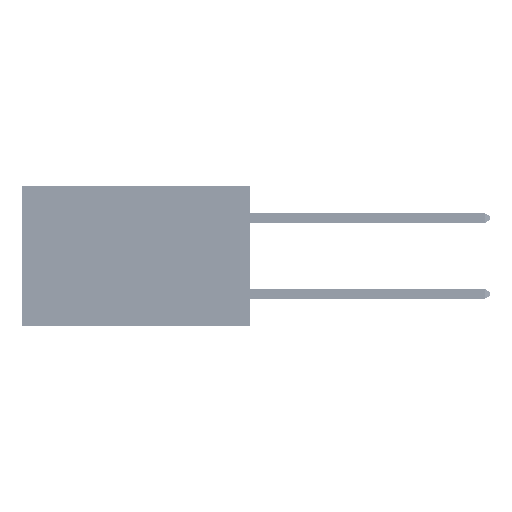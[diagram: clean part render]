
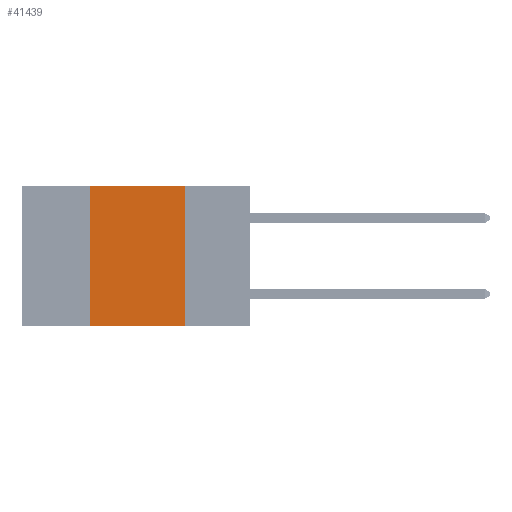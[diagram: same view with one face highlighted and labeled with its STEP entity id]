
A CAD part, left-side view. The second image highlights one B-rep face of the part: STEP entity #41439.
In plain terms, the highlighted planar face has unit normal (-1, 0, 0).
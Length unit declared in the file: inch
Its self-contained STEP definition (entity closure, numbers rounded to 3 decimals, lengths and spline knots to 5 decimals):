
#1589 = VECTOR ( 'NONE', #28482, 39.37008 ) ;
#3840 = VECTOR ( 'NONE', #15682, 39.37008 ) ;
#4211 = EDGE_CURVE ( 'NONE', #22656, #34241, #32235, .T. ) ;
#6393 = ORIENTED_EDGE ( 'NONE', *, *, #17723, .F. ) ;
#6564 = CARTESIAN_POINT ( 'NONE',  ( 0., 0.42, 0. ) ) ;
#7036 = DIRECTION ( 'NONE',  ( 1., 0., 0. ) ) ;
#7541 = ORIENTED_EDGE ( 'NONE', *, *, #4211, .T. ) ;
#10291 = EDGE_LOOP ( 'NONE', ( #6393, #43165, #33677, #7541 ) ) ;
#10614 = VECTOR ( 'NONE', #27359, 39.37008 ) ;
#14806 = CARTESIAN_POINT ( 'NONE',  ( 0., 0.6, -0.37 ) ) ;
#14842 = VECTOR ( 'NONE', #29393, 39.37008 ) ;
#15682 = DIRECTION ( 'NONE',  ( 0., -1., 0. ) ) ;
#17723 = EDGE_CURVE ( 'NONE', #29060, #34241, #45265, .T. ) ;
#19779 = CARTESIAN_POINT ( 'NONE',  ( 0., 0.42, 0. ) ) ;
#22656 = VERTEX_POINT ( 'NONE', #39769 ) ;
#24455 = CARTESIAN_POINT ( 'NONE',  ( 0., 0.6, 0. ) ) ;
#24463 = LINE ( 'NONE', #6564, #1589 ) ;
#25095 = VERTEX_POINT ( 'NONE', #19779 ) ;
#27359 = DIRECTION ( 'NONE',  ( 0., 0., -1. ) ) ;
#28482 = DIRECTION ( 'NONE',  ( 0., 0., 1. ) ) ;
#29060 = VERTEX_POINT ( 'NONE', #42988 ) ;
#29393 = DIRECTION ( 'NONE',  ( 0., -1., 0. ) ) ;
#29553 = CARTESIAN_POINT ( 'NONE',  ( 0., 0.17, -0.37 ) ) ;
#32235 = LINE ( 'NONE', #14806, #14842 ) ;
#32624 = EDGE_CURVE ( 'NONE', #25095, #29060, #41134, .T. ) ;
#33677 = ORIENTED_EDGE ( 'NONE', *, *, #39256, .F. ) ;
#34241 = VERTEX_POINT ( 'NONE', #29553 ) ;
#35774 = DIRECTION ( 'NONE',  ( 0., 0., -1. ) ) ;
#37142 = CARTESIAN_POINT ( 'NONE',  ( 0., 0.6, 0. ) ) ;
#38415 = CARTESIAN_POINT ( 'NONE',  ( 0., 0.17, 0. ) ) ;
#39245 = AXIS2_PLACEMENT_3D ( 'NONE', #24455, #7036, #35774 ) ;
#39256 = EDGE_CURVE ( 'NONE', #22656, #25095, #24463, .T. ) ;
#39769 = CARTESIAN_POINT ( 'NONE',  ( 0., 0.42, -0.37 ) ) ;
#41134 = LINE ( 'NONE', #37142, #3840 ) ;
#41439 = ADVANCED_FACE ( 'NONE', ( #42618 ), #43092, .F. ) ;
#42618 = FACE_OUTER_BOUND ( 'NONE', #10291, .T. ) ;
#42988 = CARTESIAN_POINT ( 'NONE',  ( 0., 0.17, 0. ) ) ;
#43092 = PLANE ( 'NONE',  #39245 ) ;
#43165 = ORIENTED_EDGE ( 'NONE', *, *, #32624, .F. ) ;
#45265 = LINE ( 'NONE', #38415, #10614 ) ;
